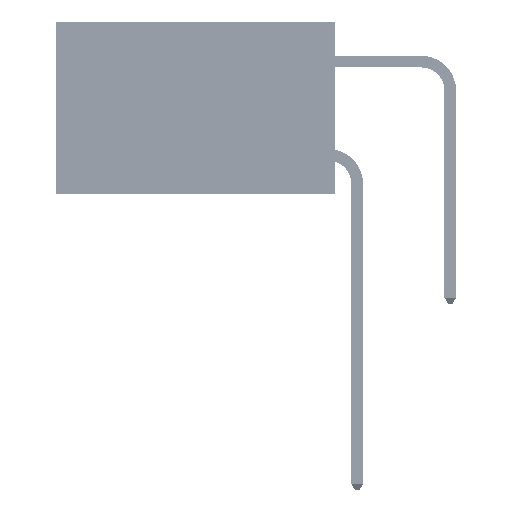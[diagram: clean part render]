
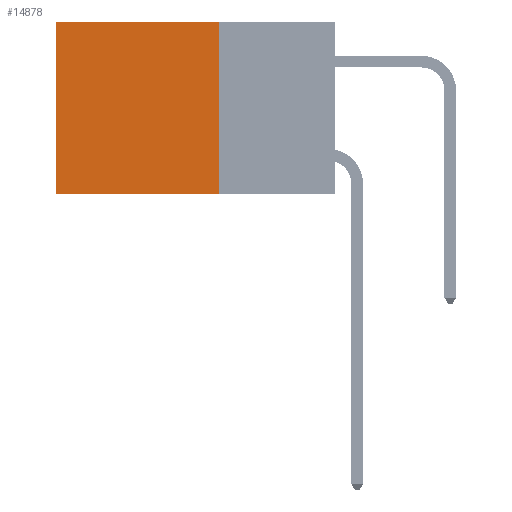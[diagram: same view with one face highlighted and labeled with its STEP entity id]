
A CAD part, left-side view. The second image highlights one B-rep face of the part: STEP entity #14878.
In plain terms, the highlighted planar face has unit normal (-1, 0, 0).
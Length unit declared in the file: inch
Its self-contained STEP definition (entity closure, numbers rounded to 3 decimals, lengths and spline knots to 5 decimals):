
#3877 = DIRECTION ( 'NONE',  ( 0., 0., -1. ) ) ;
#6249 = LINE ( 'NONE', #8900, #14982 ) ;
#8900 = CARTESIAN_POINT ( 'NONE',  ( 0.2875, 0.25, -0.37 ) ) ;
#9596 = ORIENTED_EDGE ( 'NONE', *, *, #21977, .F. ) ;
#10442 = CARTESIAN_POINT ( 'NONE',  ( 0.2875, 0.25, 0. ) ) ;
#11708 = EDGE_CURVE ( 'NONE', #46702, #45050, #22228, .T. ) ;
#13862 = CARTESIAN_POINT ( 'NONE',  ( 0.2875, 0.25, 0. ) ) ;
#14878 = ADVANCED_FACE ( 'NONE', ( #35386 ), #28533, .F. ) ;
#14982 = VECTOR ( 'NONE', #38553, 39.37008 ) ;
#15200 = CARTESIAN_POINT ( 'NONE',  ( 0.2875, 0.6, 0. ) ) ;
#15401 = CARTESIAN_POINT ( 'NONE',  ( 0.2875, 0.6, 0. ) ) ;
#15794 = VECTOR ( 'NONE', #3877, 39.37008 ) ;
#17855 = VECTOR ( 'NONE', #28845, 39.37008 ) ;
#20267 = CARTESIAN_POINT ( 'NONE',  ( 0.2875, 0.25, 0. ) ) ;
#21977 = EDGE_CURVE ( 'NONE', #45050, #37651, #6249, .T. ) ;
#22228 = LINE ( 'NONE', #20267, #37430 ) ;
#24148 = DIRECTION ( 'NONE',  ( 0., 0., -1. ) ) ;
#25014 = CARTESIAN_POINT ( 'NONE',  ( 0.2875, 0.25, 0. ) ) ;
#26006 = EDGE_CURVE ( 'NONE', #46702, #30134, #38248, .T. ) ;
#28533 = PLANE ( 'NONE',  #37692 ) ;
#28845 = DIRECTION ( 'NONE',  ( 0., 1., 0. ) ) ;
#28873 = ORIENTED_EDGE ( 'NONE', *, *, #43639, .T. ) ;
#29117 = EDGE_LOOP ( 'NONE', ( #28873, #9596, #39709, #41991 ) ) ;
#30134 = VERTEX_POINT ( 'NONE', #15200 ) ;
#35386 = FACE_OUTER_BOUND ( 'NONE', #29117, .T. ) ;
#36385 = DIRECTION ( 'NONE',  ( 0., 0., -1. ) ) ;
#37239 = CARTESIAN_POINT ( 'NONE',  ( 0.2875, 0.6, -0.37 ) ) ;
#37430 = VECTOR ( 'NONE', #24148, 39.37008 ) ;
#37651 = VERTEX_POINT ( 'NONE', #37239 ) ;
#37692 = AXIS2_PLACEMENT_3D ( 'NONE', #10442, #47805, #36385 ) ;
#38248 = LINE ( 'NONE', #13862, #17855 ) ;
#38553 = DIRECTION ( 'NONE',  ( 0., 1., 0. ) ) ;
#39178 = CARTESIAN_POINT ( 'NONE',  ( 0.2875, 0.25, -0.37 ) ) ;
#39709 = ORIENTED_EDGE ( 'NONE', *, *, #11708, .F. ) ;
#41991 = ORIENTED_EDGE ( 'NONE', *, *, #26006, .T. ) ;
#43639 = EDGE_CURVE ( 'NONE', #30134, #37651, #44393, .T. ) ;
#44393 = LINE ( 'NONE', #15401, #15794 ) ;
#45050 = VERTEX_POINT ( 'NONE', #39178 ) ;
#46702 = VERTEX_POINT ( 'NONE', #25014 ) ;
#47805 = DIRECTION ( 'NONE',  ( 1., 0., 0. ) ) ;
